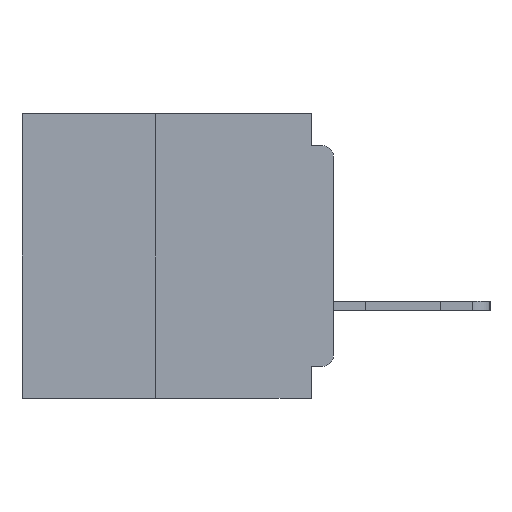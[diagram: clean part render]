
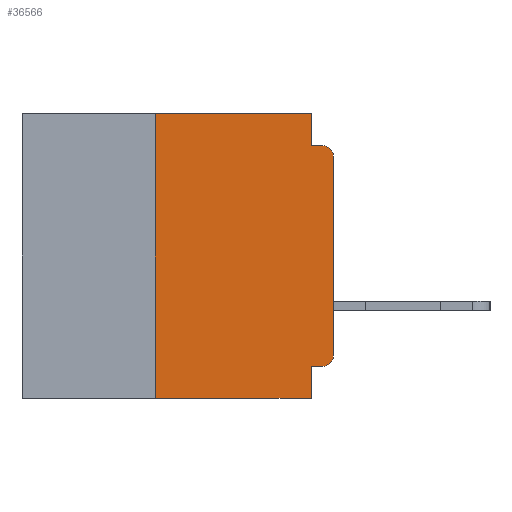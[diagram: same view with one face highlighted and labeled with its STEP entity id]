
A CAD part, left-side view. The second image highlights one B-rep face of the part: STEP entity #36566.
In plain terms, the highlighted planar face has unit normal (-1, 0, 0).
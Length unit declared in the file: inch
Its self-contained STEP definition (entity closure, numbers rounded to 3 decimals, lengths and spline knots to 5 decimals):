
#356 = VERTEX_POINT ( 'NONE', #531 ) ;
#384 = DIRECTION ( 'NONE',  ( 0., 0., -1. ) ) ;
#531 = CARTESIAN_POINT ( 'NONE',  ( 0., 0.031, -0.355 ) ) ;
#782 = VECTOR ( 'NONE', #40366, 39.37008 ) ;
#924 = EDGE_CURVE ( 'NONE', #29006, #56146, #24800, .T. ) ;
#2643 = LINE ( 'NONE', #56608, #26589 ) ;
#2708 = CARTESIAN_POINT ( 'NONE',  ( 0., 0.015, -0.34 ) ) ;
#2845 = DIRECTION ( 'NONE',  ( 0., -1., 0. ) ) ;
#3684 = CARTESIAN_POINT ( 'NONE',  ( 0., 0.015, -0.06 ) ) ;
#4177 = VERTEX_POINT ( 'NONE', #35048 ) ;
#4530 = EDGE_CURVE ( 'NONE', #58009, #34500, #27815, .T. ) ;
#6106 = EDGE_LOOP ( 'NONE', ( #9434, #37274, #54406, #50962, #18041, #26791, #43769, #25627, #16348, #46558 ) ) ;
#6372 = FACE_OUTER_BOUND ( 'NONE', #6106, .T. ) ;
#7202 = PLANE ( 'NONE',  #33968 ) ;
#7291 = DIRECTION ( 'NONE',  ( 0., 0., -1. ) ) ;
#8258 = DIRECTION ( 'NONE',  ( 0., 0., -1. ) ) ;
#8434 = VECTOR ( 'NONE', #384, 39.37008 ) ;
#9313 = VERTEX_POINT ( 'NONE', #55146 ) ;
#9421 = DIRECTION ( 'NONE',  ( 0., 1., 0. ) ) ;
#9434 = ORIENTED_EDGE ( 'NONE', *, *, #53790, .T. ) ;
#10421 = CARTESIAN_POINT ( 'NONE',  ( 0., 0., -0.045 ) ) ;
#10928 = LINE ( 'NONE', #22189, #33388 ) ;
#11174 = EDGE_CURVE ( 'NONE', #58009, #56101, #36160, .T. ) ;
#12504 = LINE ( 'NONE', #10421, #36352 ) ;
#13070 = EDGE_CURVE ( 'NONE', #34500, #29006, #2643, .T. ) ;
#13390 = DIRECTION ( 'NONE',  ( 0., 0., 1. ) ) ;
#13694 = VECTOR ( 'NONE', #56216, 39.37008 ) ;
#16294 = CARTESIAN_POINT ( 'NONE',  ( 0., 0.437, 0. ) ) ;
#16348 = ORIENTED_EDGE ( 'NONE', *, *, #24704, .F. ) ;
#17356 = VECTOR ( 'NONE', #17771, 39.37008 ) ;
#17771 = DIRECTION ( 'NONE',  ( 0., 0., 1. ) ) ;
#17833 = CARTESIAN_POINT ( 'NONE',  ( 0., 0.25, -0.4 ) ) ;
#18041 = ORIENTED_EDGE ( 'NONE', *, *, #13070, .F. ) ;
#18720 = VERTEX_POINT ( 'NONE', #36452 ) ;
#20398 = LINE ( 'NONE', #45309, #8434 ) ;
#20783 = DIRECTION ( 'NONE',  ( 0., 0., -1. ) ) ;
#22189 = CARTESIAN_POINT ( 'NONE',  ( 0., 0., 0. ) ) ;
#24289 = CARTESIAN_POINT ( 'NONE',  ( 0., 0.25, 0. ) ) ;
#24704 = EDGE_CURVE ( 'NONE', #51165, #356, #25877, .T. ) ;
#24800 = LINE ( 'NONE', #38643, #782 ) ;
#24904 = CARTESIAN_POINT ( 'NONE',  ( 0., 0.437, -0.4 ) ) ;
#25607 = EDGE_CURVE ( 'NONE', #56146, #18720, #12504, .T. ) ;
#25627 = ORIENTED_EDGE ( 'NONE', *, *, #52585, .F. ) ;
#25877 = LINE ( 'NONE', #27246, #48365 ) ;
#26589 = VECTOR ( 'NONE', #2845, 39.37008 ) ;
#26791 = ORIENTED_EDGE ( 'NONE', *, *, #4530, .F. ) ;
#27246 = CARTESIAN_POINT ( 'NONE',  ( 0., 0., -0.355 ) ) ;
#27815 = LINE ( 'NONE', #17833, #17356 ) ;
#27864 = CARTESIAN_POINT ( 'NONE',  ( 0., 0.031, -0.4 ) ) ;
#29006 = VERTEX_POINT ( 'NONE', #34118 ) ;
#32629 = CARTESIAN_POINT ( 'NONE',  ( 0., 0.031, -0.045 ) ) ;
#33388 = VECTOR ( 'NONE', #13390, 39.37008 ) ;
#33968 = AXIS2_PLACEMENT_3D ( 'NONE', #16294, #47638, #20783 ) ;
#34118 = CARTESIAN_POINT ( 'NONE',  ( 0., 0.031, 0. ) ) ;
#34229 = DIRECTION ( 'NONE',  ( -1., 0., 0. ) ) ;
#34500 = VERTEX_POINT ( 'NONE', #24289 ) ;
#35048 = CARTESIAN_POINT ( 'NONE',  ( 0., 0., -0.06 ) ) ;
#35186 = DIRECTION ( 'NONE',  ( -1., 0., 0. ) ) ;
#36160 = LINE ( 'NONE', #24904, #13694 ) ;
#36352 = VECTOR ( 'NONE', #50753, 39.37008 ) ;
#36452 = CARTESIAN_POINT ( 'NONE',  ( 0., 0.015, -0.045 ) ) ;
#36566 = ADVANCED_FACE ( 'NONE', ( #6372 ), #7202, .F. ) ;
#37274 = ORIENTED_EDGE ( 'NONE', *, *, #37826, .T. ) ;
#37348 = CARTESIAN_POINT ( 'NONE',  ( 0., 0.25, -0.4 ) ) ;
#37795 = CIRCLE ( 'NONE', #53438, 0.015 ) ;
#37826 = EDGE_CURVE ( 'NONE', #4177, #18720, #37795, .T. ) ;
#38643 = CARTESIAN_POINT ( 'NONE',  ( 0., 0.031, 0. ) ) ;
#40366 = DIRECTION ( 'NONE',  ( 0., 0., -1. ) ) ;
#42586 = CIRCLE ( 'NONE', #45517, 0.015 ) ;
#43769 = ORIENTED_EDGE ( 'NONE', *, *, #11174, .T. ) ;
#44309 = CARTESIAN_POINT ( 'NONE',  ( 0., 0.015, -0.355 ) ) ;
#45185 = EDGE_CURVE ( 'NONE', #51165, #9313, #42586, .T. ) ;
#45309 = CARTESIAN_POINT ( 'NONE',  ( 0., 0.031, -0.4 ) ) ;
#45517 = AXIS2_PLACEMENT_3D ( 'NONE', #2708, #34229, #7291 ) ;
#46558 = ORIENTED_EDGE ( 'NONE', *, *, #45185, .T. ) ;
#47638 = DIRECTION ( 'NONE',  ( 1., 0., 0. ) ) ;
#48365 = VECTOR ( 'NONE', #9421, 39.37008 ) ;
#50753 = DIRECTION ( 'NONE',  ( 0., -1., 0. ) ) ;
#50962 = ORIENTED_EDGE ( 'NONE', *, *, #924, .F. ) ;
#51165 = VERTEX_POINT ( 'NONE', #44309 ) ;
#52585 = EDGE_CURVE ( 'NONE', #356, #56101, #20398, .T. ) ;
#53438 = AXIS2_PLACEMENT_3D ( 'NONE', #3684, #35186, #8258 ) ;
#53790 = EDGE_CURVE ( 'NONE', #9313, #4177, #10928, .T. ) ;
#54406 = ORIENTED_EDGE ( 'NONE', *, *, #25607, .F. ) ;
#55146 = CARTESIAN_POINT ( 'NONE',  ( 0., 0., -0.34 ) ) ;
#56101 = VERTEX_POINT ( 'NONE', #27864 ) ;
#56146 = VERTEX_POINT ( 'NONE', #32629 ) ;
#56216 = DIRECTION ( 'NONE',  ( 0., -1., 0. ) ) ;
#56608 = CARTESIAN_POINT ( 'NONE',  ( 0., 0.437, 0. ) ) ;
#58009 = VERTEX_POINT ( 'NONE', #37348 ) ;
